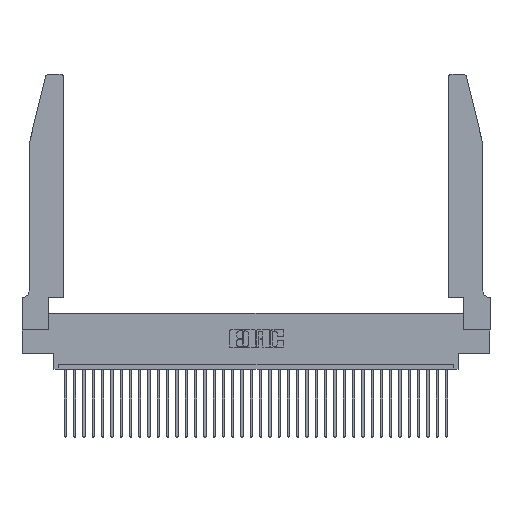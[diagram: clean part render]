
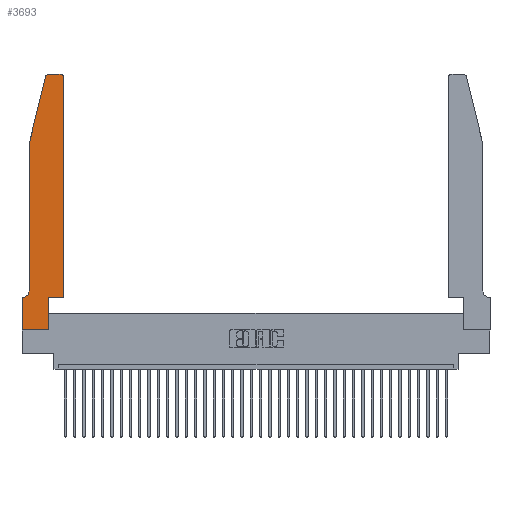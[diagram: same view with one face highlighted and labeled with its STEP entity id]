
A CAD part, top view. The second image highlights one B-rep face of the part: STEP entity #3693.
In plain terms, the highlighted planar face has unit normal (0, 0, 1).
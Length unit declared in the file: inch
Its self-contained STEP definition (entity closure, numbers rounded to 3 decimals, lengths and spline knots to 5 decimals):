
#614 = DIRECTION ( 'NONE',  ( -1., 0., 0. ) ) ;
#797 = VERTEX_POINT ( 'NONE', #25447 ) ;
#1316 = ORIENTED_EDGE ( 'NONE', *, *, #33421, .T. ) ;
#1554 = LINE ( 'NONE', #30261, #13917 ) ;
#2243 = EDGE_CURVE ( 'NONE', #21503, #14206, #32250, .T. ) ;
#2354 = CARTESIAN_POINT ( 'NONE',  ( 0.0055, 0.42, 0.37 ) ) ;
#2520 = CARTESIAN_POINT ( 'NONE',  ( 0.4505, 0.35, 0.37 ) ) ;
#3308 = DIRECTION ( 'NONE',  ( -1., 0., 0. ) ) ;
#3616 = LINE ( 'NONE', #29835, #7229 ) ;
#3693 = ADVANCED_FACE ( 'NONE', ( #12348 ), #18017, .T. ) ;
#3828 = CARTESIAN_POINT ( 'NONE',  ( 0.2605, 2.75, 0.37 ) ) ;
#3879 = DIRECTION ( 'NONE',  ( 1., 0., 0. ) ) ;
#4108 = VECTOR ( 'NONE', #8743, 39.37008 ) ;
#4242 = CARTESIAN_POINT ( 'NONE',  ( 0.4505, 0.35, 0.37 ) ) ;
#4501 = CARTESIAN_POINT ( 'NONE',  ( 0.2865, 0.35, 0.37 ) ) ;
#5534 = CIRCLE ( 'NONE', #13432, 0.07 ) ;
#6505 = DIRECTION ( 'NONE',  ( 0., 0., 1. ) ) ;
#7124 = VERTEX_POINT ( 'NONE', #24832 ) ;
#7229 = VECTOR ( 'NONE', #32662, 39.37008 ) ;
#7432 = CARTESIAN_POINT ( 'NONE',  ( 0.4505, 0.35, 0.37 ) ) ;
#7603 = DIRECTION ( 'NONE',  ( 0., -1., 0. ) ) ;
#7985 = DIRECTION ( 'NONE',  ( 1., 0., 0. ) ) ;
#8307 = VERTEX_POINT ( 'NONE', #11482 ) ;
#8372 = LINE ( 'NONE', #10470, #29078 ) ;
#8523 = EDGE_CURVE ( 'NONE', #797, #8307, #3616, .T. ) ;
#8743 = DIRECTION ( 'NONE',  ( 0., -1., 0. ) ) ;
#10470 = CARTESIAN_POINT ( 'NONE',  ( 0.0755, 2., 0.37 ) ) ;
#10515 = VECTOR ( 'NONE', #3308, 39.37008 ) ;
#11383 = ORIENTED_EDGE ( 'NONE', *, *, #15817, .T. ) ;
#11482 = CARTESIAN_POINT ( 'NONE',  ( 0.2865, 0., 0.37 ) ) ;
#11824 = VERTEX_POINT ( 'NONE', #13376 ) ;
#11888 = ORIENTED_EDGE ( 'NONE', *, *, #8523, .T. ) ;
#12348 = FACE_OUTER_BOUND ( 'NONE', #35824, .T. ) ;
#13108 = DIRECTION ( 'NONE',  ( 0., 1., 0. ) ) ;
#13129 = CIRCLE ( 'NONE', #30290, 0.03 ) ;
#13145 = CARTESIAN_POINT ( 'NONE',  ( 0., 0.35, 0.37 ) ) ;
#13200 = ORIENTED_EDGE ( 'NONE', *, *, #36020, .T. ) ;
#13205 = EDGE_CURVE ( 'NONE', #7124, #35436, #23180, .T. ) ;
#13376 = CARTESIAN_POINT ( 'NONE',  ( 0.0755, 2., 0.37 ) ) ;
#13432 = AXIS2_PLACEMENT_3D ( 'NONE', #2354, #27999, #13946 ) ;
#13632 = CARTESIAN_POINT ( 'NONE',  ( 0.4505, 2.72, 0.37 ) ) ;
#13917 = VECTOR ( 'NONE', #7603, 39.37008 ) ;
#13946 = DIRECTION ( 'NONE',  ( -1., 0., 0. ) ) ;
#14206 = VERTEX_POINT ( 'NONE', #2520 ) ;
#14687 = LINE ( 'NONE', #33899, #4108 ) ;
#15817 = EDGE_CURVE ( 'NONE', #8307, #21503, #32373, .T. ) ;
#16793 = LINE ( 'NONE', #26256, #10515 ) ;
#17214 = EDGE_CURVE ( 'NONE', #14206, #32615, #32259, .T. ) ;
#17265 = EDGE_CURVE ( 'NONE', #35436, #28367, #29193, .T. ) ;
#17463 = VECTOR ( 'NONE', #35814, 39.37008 ) ;
#17832 = AXIS2_PLACEMENT_3D ( 'NONE', #20706, #6505, #3879 ) ;
#18017 = PLANE ( 'NONE',  #17832 ) ;
#19062 = DIRECTION ( 'NONE',  ( -0.239, -0.971, 0. ) ) ;
#19158 = CARTESIAN_POINT ( 'NONE',  ( 0.4205, 2.72, 0.37 ) ) ;
#19310 = DIRECTION ( 'NONE',  ( 0., 0., 1. ) ) ;
#19406 = DIRECTION ( 'NONE',  ( 0., 0., 1. ) ) ;
#19707 = ORIENTED_EDGE ( 'NONE', *, *, #17265, .T. ) ;
#19834 = EDGE_CURVE ( 'NONE', #23793, #32406, #16793, .T. ) ;
#20706 = CARTESIAN_POINT ( 'NONE',  ( 0., 0.35, 0.37 ) ) ;
#21165 = ORIENTED_EDGE ( 'NONE', *, *, #2243, .T. ) ;
#21503 = VERTEX_POINT ( 'NONE', #24878 ) ;
#21913 = VECTOR ( 'NONE', #614, 39.37008 ) ;
#23180 = LINE ( 'NONE', #3828, #21913 ) ;
#23200 = ORIENTED_EDGE ( 'NONE', *, *, #35513, .T. ) ;
#23793 = VERTEX_POINT ( 'NONE', #35586 ) ;
#24832 = CARTESIAN_POINT ( 'NONE',  ( 0.4205, 2.75, 0.37 ) ) ;
#24878 = CARTESIAN_POINT ( 'NONE',  ( 0.2865, 0.35, 0.37 ) ) ;
#25133 = ORIENTED_EDGE ( 'NONE', *, *, #17214, .T. ) ;
#25402 = EDGE_CURVE ( 'NONE', #32615, #7124, #13129, .T. ) ;
#25447 = CARTESIAN_POINT ( 'NONE',  ( 0., 0., 0.37 ) ) ;
#25776 = ORIENTED_EDGE ( 'NONE', *, *, #19834, .T. ) ;
#26256 = CARTESIAN_POINT ( 'NONE',  ( 0.0755, 0.35, 0.37 ) ) ;
#27041 = VECTOR ( 'NONE', #35301, 39.37008 ) ;
#27081 = ORIENTED_EDGE ( 'NONE', *, *, #25402, .T. ) ;
#27999 = DIRECTION ( 'NONE',  ( 0., 0., -1. ) ) ;
#28336 = VERTEX_POINT ( 'NONE', #32625 ) ;
#28367 = VERTEX_POINT ( 'NONE', #35230 ) ;
#29078 = VECTOR ( 'NONE', #19062, 39.37008 ) ;
#29193 = CIRCLE ( 'NONE', #34815, 0.03 ) ;
#29835 = CARTESIAN_POINT ( 'NONE',  ( 0., 0., 0.37 ) ) ;
#30060 = CARTESIAN_POINT ( 'NONE',  ( 0.284, 2.72, 0.37 ) ) ;
#30090 = VECTOR ( 'NONE', #13108, 39.37008 ) ;
#30261 = CARTESIAN_POINT ( 'NONE',  ( 0., 0., 0.37 ) ) ;
#30290 = AXIS2_PLACEMENT_3D ( 'NONE', #19158, #19406, #7985 ) ;
#30291 = EDGE_CURVE ( 'NONE', #28336, #23793, #5534, .T. ) ;
#31238 = ORIENTED_EDGE ( 'NONE', *, *, #13205, .T. ) ;
#32250 = LINE ( 'NONE', #4242, #27041 ) ;
#32259 = LINE ( 'NONE', #7432, #30090 ) ;
#32373 = LINE ( 'NONE', #4501, #17463 ) ;
#32406 = VERTEX_POINT ( 'NONE', #13145 ) ;
#32615 = VERTEX_POINT ( 'NONE', #13632 ) ;
#32625 = CARTESIAN_POINT ( 'NONE',  ( 0.0755, 0.42, 0.37 ) ) ;
#32662 = DIRECTION ( 'NONE',  ( 1., 0., 0. ) ) ;
#33421 = EDGE_CURVE ( 'NONE', #11824, #28336, #14687, .T. ) ;
#33657 = ORIENTED_EDGE ( 'NONE', *, *, #30291, .T. ) ;
#33899 = CARTESIAN_POINT ( 'NONE',  ( 0.0755, 2., 0.37 ) ) ;
#34815 = AXIS2_PLACEMENT_3D ( 'NONE', #30060, #19310, #35887 ) ;
#35230 = CARTESIAN_POINT ( 'NONE',  ( 0.25487, 2.72718, 0.37 ) ) ;
#35301 = DIRECTION ( 'NONE',  ( 1., 0., 0. ) ) ;
#35436 = VERTEX_POINT ( 'NONE', #36252 ) ;
#35513 = EDGE_CURVE ( 'NONE', #28367, #11824, #8372, .T. ) ;
#35586 = CARTESIAN_POINT ( 'NONE',  ( 0.0055, 0.35, 0.37 ) ) ;
#35814 = DIRECTION ( 'NONE',  ( 0., 1., 0. ) ) ;
#35824 = EDGE_LOOP ( 'NONE', ( #31238, #19707, #23200, #1316, #33657, #25776, #13200, #11888, #11383, #21165, #25133, #27081 ) ) ;
#35887 = DIRECTION ( 'NONE',  ( 1., 0., 0. ) ) ;
#36020 = EDGE_CURVE ( 'NONE', #32406, #797, #1554, .T. ) ;
#36252 = CARTESIAN_POINT ( 'NONE',  ( 0.284, 2.75, 0.37 ) ) ;
